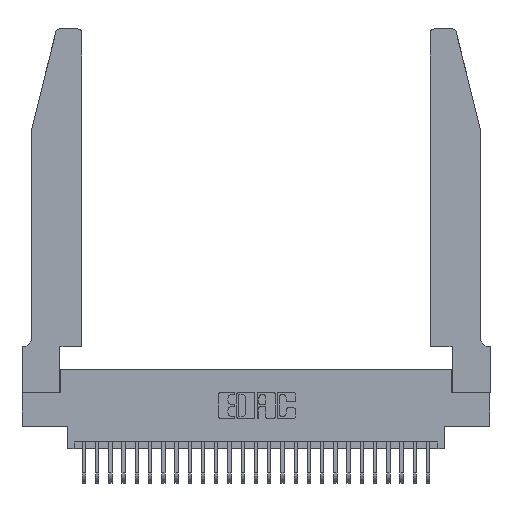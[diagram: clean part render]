
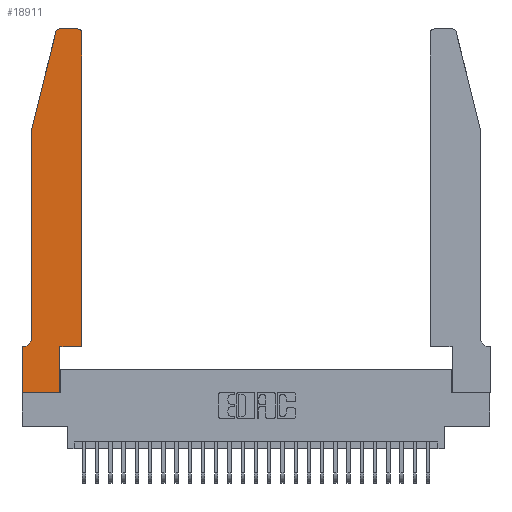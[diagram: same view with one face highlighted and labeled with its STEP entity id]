
A CAD part, top view. The second image highlights one B-rep face of the part: STEP entity #18911.
In plain terms, the highlighted planar face has unit normal (0, 0, 1).
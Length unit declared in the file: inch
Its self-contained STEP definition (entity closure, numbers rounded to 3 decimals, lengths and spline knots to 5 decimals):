
#376 = ORIENTED_EDGE ( 'NONE', *, *, #26838, .T. ) ;
#379 = AXIS2_PLACEMENT_3D ( 'NONE', #11876, #26568, #13971 ) ;
#413 = CARTESIAN_POINT ( 'NONE',  ( 0.2865, 0.35, 0.37 ) ) ;
#546 = VERTEX_POINT ( 'NONE', #9251 ) ;
#828 = DIRECTION ( 'NONE',  ( 0., 0., 1. ) ) ;
#850 = LINE ( 'NONE', #26084, #5870 ) ;
#1368 = LINE ( 'NONE', #1619, #25466 ) ;
#1619 = CARTESIAN_POINT ( 'NONE',  ( 0.0755, 0.35, 0.37 ) ) ;
#2402 = VERTEX_POINT ( 'NONE', #12216 ) ;
#2842 = CIRCLE ( 'NONE', #17569, 0.07 ) ;
#3233 = EDGE_CURVE ( 'NONE', #21981, #6892, #13003, .T. ) ;
#3544 = CARTESIAN_POINT ( 'NONE',  ( 0., 0., 0.37 ) ) ;
#3668 = CARTESIAN_POINT ( 'NONE',  ( 0.4505, 0.35, 0.37 ) ) ;
#3787 = ORIENTED_EDGE ( 'NONE', *, *, #17572, .T. ) ;
#3800 = DIRECTION ( 'NONE',  ( -1., 0., 0. ) ) ;
#4389 = EDGE_CURVE ( 'NONE', #18777, #21200, #24459, .T. ) ;
#4768 = ORIENTED_EDGE ( 'NONE', *, *, #18521, .T. ) ;
#5415 = AXIS2_PLACEMENT_3D ( 'NONE', #13520, #828, #15606 ) ;
#5870 = VECTOR ( 'NONE', #13518, 39.37008 ) ;
#6419 = EDGE_CURVE ( 'NONE', #20255, #18777, #12830, .T. ) ;
#6773 = ORIENTED_EDGE ( 'NONE', *, *, #27122, .T. ) ;
#6892 = VERTEX_POINT ( 'NONE', #15513 ) ;
#6920 = EDGE_CURVE ( 'NONE', #21605, #546, #850, .T. ) ;
#6983 = DIRECTION ( 'NONE',  ( 1., 0., 0. ) ) ;
#8088 = VECTOR ( 'NONE', #6983, 39.37008 ) ;
#8384 = CIRCLE ( 'NONE', #379, 0.03 ) ;
#8503 = DIRECTION ( 'NONE',  ( 0., -1., 0. ) ) ;
#8872 = CARTESIAN_POINT ( 'NONE',  ( 0.4505, 2.72, 0.37 ) ) ;
#9251 = CARTESIAN_POINT ( 'NONE',  ( 0.0755, 0.42, 0.37 ) ) ;
#9326 = PLANE ( 'NONE',  #17660 ) ;
#9558 = VECTOR ( 'NONE', #12209, 39.37008 ) ;
#9596 = ORIENTED_EDGE ( 'NONE', *, *, #4389, .T. ) ;
#10356 = VECTOR ( 'NONE', #23703, 39.37008 ) ;
#10609 = CARTESIAN_POINT ( 'NONE',  ( 0., 0., 0.37 ) ) ;
#11008 = VERTEX_POINT ( 'NONE', #11532 ) ;
#11017 = EDGE_CURVE ( 'NONE', #14807, #21605, #23692, .T. ) ;
#11018 = LINE ( 'NONE', #413, #10356 ) ;
#11444 = CARTESIAN_POINT ( 'NONE',  ( 0., 0.35, 0.37 ) ) ;
#11532 = CARTESIAN_POINT ( 'NONE',  ( 0.2865, 0.35, 0.37 ) ) ;
#11562 = CARTESIAN_POINT ( 'NONE',  ( 0.0055, 0.42, 0.37 ) ) ;
#11876 = CARTESIAN_POINT ( 'NONE',  ( 0.284, 2.72, 0.37 ) ) ;
#11895 = ORIENTED_EDGE ( 'NONE', *, *, #26212, .T. ) ;
#12209 = DIRECTION ( 'NONE',  ( -1., 0., 0. ) ) ;
#12216 = CARTESIAN_POINT ( 'NONE',  ( 0.0055, 0.35, 0.37 ) ) ;
#12830 = LINE ( 'NONE', #3668, #19042 ) ;
#13003 = LINE ( 'NONE', #10609, #23548 ) ;
#13324 = CARTESIAN_POINT ( 'NONE',  ( 0.4505, 0.35, 0.37 ) ) ;
#13518 = DIRECTION ( 'NONE',  ( 0., -1., 0. ) ) ;
#13520 = CARTESIAN_POINT ( 'NONE',  ( 0.4205, 2.72, 0.37 ) ) ;
#13556 = DIRECTION ( 'NONE',  ( 1., 0., 0. ) ) ;
#13641 = CARTESIAN_POINT ( 'NONE',  ( 0.0755, 2., 0.37 ) ) ;
#13671 = DIRECTION ( 'NONE',  ( -1., 0., 0. ) ) ;
#13971 = DIRECTION ( 'NONE',  ( 1., 0., 0. ) ) ;
#13976 = EDGE_CURVE ( 'NONE', #21458, #14807, #8384, .T. ) ;
#14450 = VECTOR ( 'NONE', #19887, 39.37008 ) ;
#14807 = VERTEX_POINT ( 'NONE', #16963 ) ;
#15041 = ORIENTED_EDGE ( 'NONE', *, *, #3233, .T. ) ;
#15100 = VECTOR ( 'NONE', #24518, 39.37008 ) ;
#15120 = CARTESIAN_POINT ( 'NONE',  ( 0.284, 2.75, 0.37 ) ) ;
#15513 = CARTESIAN_POINT ( 'NONE',  ( 0., 0., 0.37 ) ) ;
#15606 = DIRECTION ( 'NONE',  ( 1., 0., 0. ) ) ;
#15608 = ORIENTED_EDGE ( 'NONE', *, *, #13976, .T. ) ;
#16963 = CARTESIAN_POINT ( 'NONE',  ( 0.25487, 2.72718, 0.37 ) ) ;
#17569 = AXIS2_PLACEMENT_3D ( 'NONE', #11562, #26241, #13671 ) ;
#17572 = EDGE_CURVE ( 'NONE', #21200, #21458, #20769, .T. ) ;
#17660 = AXIS2_PLACEMENT_3D ( 'NONE', #11444, #26120, #13556 ) ;
#18521 = EDGE_CURVE ( 'NONE', #6892, #26031, #25635, .T. ) ;
#18762 = CARTESIAN_POINT ( 'NONE',  ( 0., 0.35, 0.37 ) ) ;
#18777 = VERTEX_POINT ( 'NONE', #8872 ) ;
#18911 = ADVANCED_FACE ( 'NONE', ( #21358 ), #9326, .T. ) ;
#19042 = VECTOR ( 'NONE', #20492, 39.37008 ) ;
#19252 = LINE ( 'NONE', #13324, #8088 ) ;
#19347 = EDGE_LOOP ( 'NONE', ( #3787, #15608, #22821, #25218, #21817, #6773, #15041, #4768, #376, #11895, #20546, #9596 ) ) ;
#19887 = DIRECTION ( 'NONE',  ( -0.239, -0.971, 0. ) ) ;
#20255 = VERTEX_POINT ( 'NONE', #22520 ) ;
#20492 = DIRECTION ( 'NONE',  ( 0., 1., 0. ) ) ;
#20546 = ORIENTED_EDGE ( 'NONE', *, *, #6419, .T. ) ;
#20769 = LINE ( 'NONE', #22698, #9558 ) ;
#21200 = VERTEX_POINT ( 'NONE', #26802 ) ;
#21358 = FACE_OUTER_BOUND ( 'NONE', #19347, .T. ) ;
#21458 = VERTEX_POINT ( 'NONE', #15120 ) ;
#21605 = VERTEX_POINT ( 'NONE', #26130 ) ;
#21817 = ORIENTED_EDGE ( 'NONE', *, *, #25525, .T. ) ;
#21981 = VERTEX_POINT ( 'NONE', #18762 ) ;
#22520 = CARTESIAN_POINT ( 'NONE',  ( 0.4505, 0.35, 0.37 ) ) ;
#22698 = CARTESIAN_POINT ( 'NONE',  ( 0.2605, 2.75, 0.37 ) ) ;
#22821 = ORIENTED_EDGE ( 'NONE', *, *, #11017, .T. ) ;
#23548 = VECTOR ( 'NONE', #8503, 39.37008 ) ;
#23692 = LINE ( 'NONE', #13641, #14450 ) ;
#23703 = DIRECTION ( 'NONE',  ( 0., 1., 0. ) ) ;
#24459 = CIRCLE ( 'NONE', #5415, 0.03 ) ;
#24518 = DIRECTION ( 'NONE',  ( 1., 0., 0. ) ) ;
#25218 = ORIENTED_EDGE ( 'NONE', *, *, #6920, .T. ) ;
#25466 = VECTOR ( 'NONE', #3800, 39.37008 ) ;
#25525 = EDGE_CURVE ( 'NONE', #546, #2402, #2842, .T. ) ;
#25635 = LINE ( 'NONE', #3544, #15100 ) ;
#25778 = CARTESIAN_POINT ( 'NONE',  ( 0.2865, 0., 0.37 ) ) ;
#26031 = VERTEX_POINT ( 'NONE', #25778 ) ;
#26084 = CARTESIAN_POINT ( 'NONE',  ( 0.0755, 2., 0.37 ) ) ;
#26120 = DIRECTION ( 'NONE',  ( 0., 0., 1. ) ) ;
#26130 = CARTESIAN_POINT ( 'NONE',  ( 0.0755, 2., 0.37 ) ) ;
#26212 = EDGE_CURVE ( 'NONE', #11008, #20255, #19252, .T. ) ;
#26241 = DIRECTION ( 'NONE',  ( 0., 0., -1. ) ) ;
#26568 = DIRECTION ( 'NONE',  ( 0., 0., 1. ) ) ;
#26802 = CARTESIAN_POINT ( 'NONE',  ( 0.4205, 2.75, 0.37 ) ) ;
#26838 = EDGE_CURVE ( 'NONE', #26031, #11008, #11018, .T. ) ;
#27122 = EDGE_CURVE ( 'NONE', #2402, #21981, #1368, .T. ) ;
